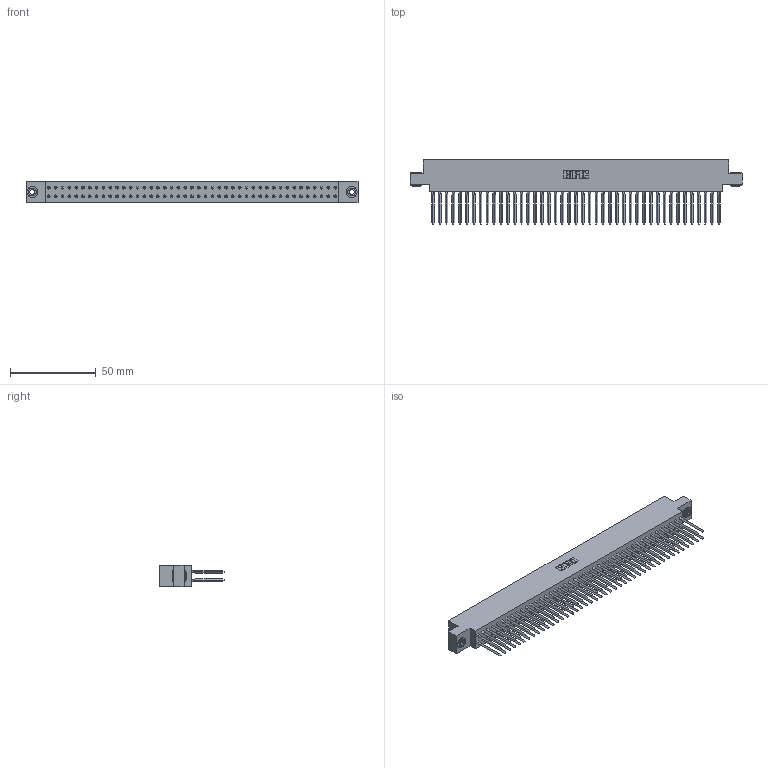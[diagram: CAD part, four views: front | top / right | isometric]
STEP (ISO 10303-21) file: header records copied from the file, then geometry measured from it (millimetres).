
FILE_DESCRIPTION (( 'STEP AP203' ), '1' );
FILE_NAME ('317-086-542-803.STEP', '2020-02-28T10:36:33', ( '' ), ( '' ), 'SwSTEP 2.0', 'SolidWorks 2016', '' );
FILE_SCHEMA (( 'CONFIG_CONTROL_DESIGN' ));
Length unit declared in the file: inch
Products named in the file (4): 345-250-002_345-250-002-102; 317-086-542-803; 317 Part_.156 Dia - TH; 317-290-003_542
Assembly tree (89 placements, depth 2):
  317-086-542-803
    317 Part_.156 Dia - TH
    317-290-003_542  x86
    345-250-002_345-250-002-102  x2
Bounding box: 193.09 x 37.34 x 12.7 mm (x, y, z)
Volume: 31669 mm3; surface area: 44286.9 mm2
Topology: 89 solids, 89 shells, 5042 faces, 14111 edges, 9002 vertices
Faces by surface type: plane 4024, cylinder 666, bspline 344, cone 8
Entity records: 61684 total; most frequent: CARTESIAN_POINT 10980, ORIENTED_EDGE 10636, DIRECTION 8984, EDGE_CURVE 5318, LINE 5124, VECTOR 5124, VERTEX_POINT 3538, AXIS2_PLACEMENT_3D 1930
